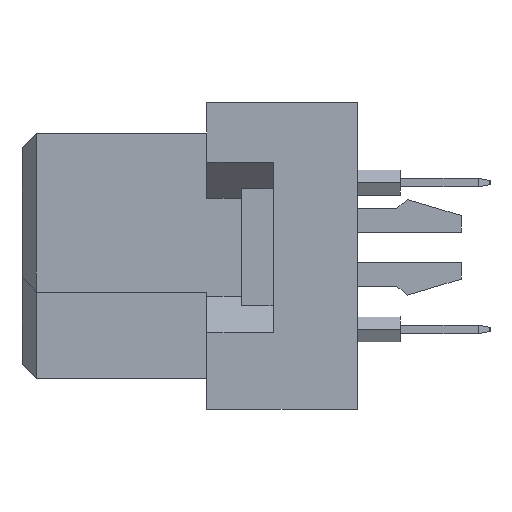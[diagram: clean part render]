
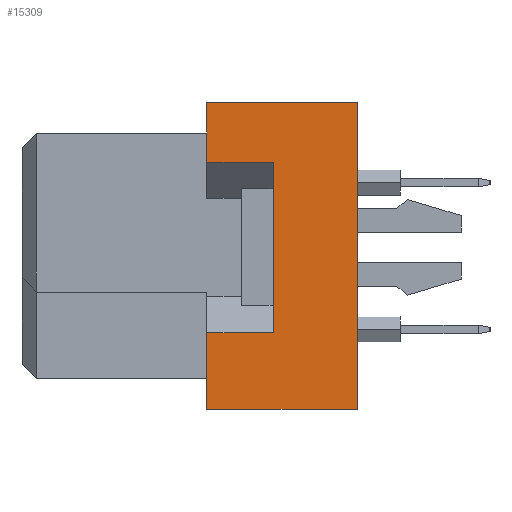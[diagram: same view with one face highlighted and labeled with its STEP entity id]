
A CAD part, left-side view. The second image highlights one B-rep face of the part: STEP entity #15309.
In plain terms, the highlighted planar face has unit normal (-1, 0, 0).
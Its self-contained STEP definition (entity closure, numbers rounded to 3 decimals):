
#24 = DIRECTION ( 'NONE',  ( -1., 0., 0. ) ) ;
#823 = VECTOR ( 'NONE', #4692, 1000. ) ;
#1492 = DIRECTION ( 'NONE',  ( 0., 0., 1. ) ) ;
#2024 = LINE ( 'NONE', #39699, #823 ) ;
#2317 = VERTEX_POINT ( 'NONE', #30488 ) ;
#3514 = CARTESIAN_POINT ( 'NONE',  ( -47.5, -8.7, 3.25 ) ) ;
#4692 = DIRECTION ( 'NONE',  ( 0., 0., 1. ) ) ;
#4921 = CARTESIAN_POINT ( 'NONE',  ( -47.5, -6.4, -5.3 ) ) ;
#6401 = DIRECTION ( 'NONE',  ( 0., 0., 1. ) ) ;
#6492 = LINE ( 'NONE', #10204, #23217 ) ;
#7153 = EDGE_CURVE ( 'NONE', #2317, #19050, #7681, .T. ) ;
#7681 = LINE ( 'NONE', #29672, #23260 ) ;
#8318 = CARTESIAN_POINT ( 'NONE',  ( -47.5, -6.4, 3.25 ) ) ;
#9268 = LINE ( 'NONE', #3514, #16038 ) ;
#9281 = FACE_OUTER_BOUND ( 'NONE', #35739, .T. ) ;
#9531 = CARTESIAN_POINT ( 'NONE',  ( -47.5, -11.6, -5.3 ) ) ;
#9791 = DIRECTION ( 'NONE',  ( 0., 1., 0. ) ) ;
#10204 = CARTESIAN_POINT ( 'NONE',  ( -47.5, -11.6, 5.3 ) ) ;
#12585 = CARTESIAN_POINT ( 'NONE',  ( -47.5, -8.7, -2.65 ) ) ;
#12815 = LINE ( 'NONE', #9531, #34802 ) ;
#12835 = LINE ( 'NONE', #38730, #36269 ) ;
#13454 = VERTEX_POINT ( 'NONE', #8318 ) ;
#13722 = EDGE_CURVE ( 'NONE', #22229, #27780, #12835, .T. ) ;
#13938 = ORIENTED_EDGE ( 'NONE', *, *, #13722, .F. ) ;
#14341 = ORIENTED_EDGE ( 'NONE', *, *, #21141, .T. ) ;
#14548 = CARTESIAN_POINT ( 'NONE',  ( -47.5, -11.6, 5.3 ) ) ;
#15309 = ADVANCED_FACE ( 'NONE', ( #9281 ), #34391, .T. ) ;
#15900 = DIRECTION ( 'NONE',  ( 0., 0., 1. ) ) ;
#16038 = VECTOR ( 'NONE', #21813, 1000. ) ;
#16058 = EDGE_CURVE ( 'NONE', #13454, #25899, #2024, .T. ) ;
#16655 = VECTOR ( 'NONE', #31189, 1000. ) ;
#17606 = ORIENTED_EDGE ( 'NONE', *, *, #7153, .T. ) ;
#18760 = CARTESIAN_POINT ( 'NONE',  ( -47.5, -11.6, 5.3 ) ) ;
#19050 = VERTEX_POINT ( 'NONE', #14548 ) ;
#19164 = LINE ( 'NONE', #12585, #30345 ) ;
#19519 = ORIENTED_EDGE ( 'NONE', *, *, #37297, .F. ) ;
#19863 = VERTEX_POINT ( 'NONE', #25614 ) ;
#20526 = CARTESIAN_POINT ( 'NONE',  ( -47.5, -6.4, 5.3 ) ) ;
#21141 = EDGE_CURVE ( 'NONE', #19050, #25899, #6492, .T. ) ;
#21813 = DIRECTION ( 'NONE',  ( 0., 1., 0. ) ) ;
#21957 = EDGE_CURVE ( 'NONE', #31841, #13454, #9268, .T. ) ;
#22229 = VERTEX_POINT ( 'NONE', #4921 ) ;
#22750 = LINE ( 'NONE', #38379, #16655 ) ;
#23217 = VECTOR ( 'NONE', #9791, 1000. ) ;
#23260 = VECTOR ( 'NONE', #1492, 1000. ) ;
#25115 = CARTESIAN_POINT ( 'NONE',  ( -47.5, -8.7, 3.25 ) ) ;
#25368 = DIRECTION ( 'NONE',  ( 0., 1., 0. ) ) ;
#25614 = CARTESIAN_POINT ( 'NONE',  ( -47.5, -8.7, -2.65 ) ) ;
#25899 = VERTEX_POINT ( 'NONE', #20526 ) ;
#27606 = ORIENTED_EDGE ( 'NONE', *, *, #29995, .F. ) ;
#27780 = VERTEX_POINT ( 'NONE', #39739 ) ;
#27893 = ORIENTED_EDGE ( 'NONE', *, *, #21957, .F. ) ;
#28853 = DIRECTION ( 'NONE',  ( 0., 1., 0. ) ) ;
#29062 = ORIENTED_EDGE ( 'NONE', *, *, #16058, .F. ) ;
#29672 = CARTESIAN_POINT ( 'NONE',  ( -47.5, -11.6, 5.3 ) ) ;
#29995 = EDGE_CURVE ( 'NONE', #19863, #31841, #22750, .T. ) ;
#30345 = VECTOR ( 'NONE', #28853, 1000. ) ;
#30488 = CARTESIAN_POINT ( 'NONE',  ( -47.5, -11.6, -5.3 ) ) ;
#31189 = DIRECTION ( 'NONE',  ( 0., 0., 1. ) ) ;
#31841 = VERTEX_POINT ( 'NONE', #25115 ) ;
#34185 = ORIENTED_EDGE ( 'NONE', *, *, #40045, .T. ) ;
#34391 = PLANE ( 'NONE',  #35597 ) ;
#34802 = VECTOR ( 'NONE', #25368, 1000. ) ;
#35597 = AXIS2_PLACEMENT_3D ( 'NONE', #18760, #24, #6401 ) ;
#35739 = EDGE_LOOP ( 'NONE', ( #34185, #13938, #19519, #17606, #14341, #29062, #27893, #27606 ) ) ;
#36269 = VECTOR ( 'NONE', #15900, 1000. ) ;
#37297 = EDGE_CURVE ( 'NONE', #2317, #22229, #12815, .T. ) ;
#38379 = CARTESIAN_POINT ( 'NONE',  ( -47.5, -8.7, -2.65 ) ) ;
#38730 = CARTESIAN_POINT ( 'NONE',  ( -47.5, -6.4, -5.3 ) ) ;
#39699 = CARTESIAN_POINT ( 'NONE',  ( -47.5, -6.4, -5.3 ) ) ;
#39739 = CARTESIAN_POINT ( 'NONE',  ( -47.5, -6.4, -2.65 ) ) ;
#40045 = EDGE_CURVE ( 'NONE', #19863, #27780, #19164, .T. ) ;
